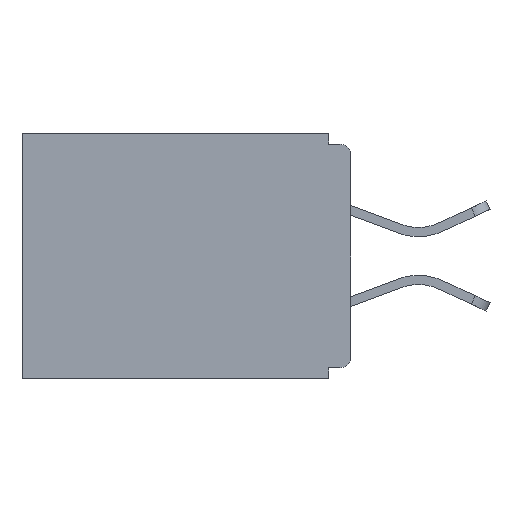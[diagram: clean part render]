
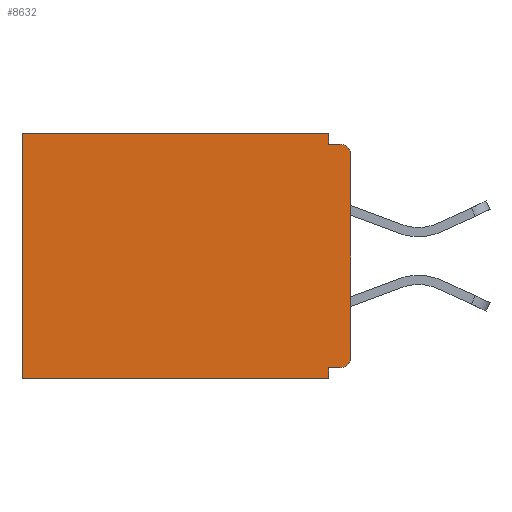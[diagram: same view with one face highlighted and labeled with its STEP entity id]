
A CAD part, left-side view. The second image highlights one B-rep face of the part: STEP entity #8632.
In plain terms, the highlighted planar face has unit normal (-1, 0, 0).
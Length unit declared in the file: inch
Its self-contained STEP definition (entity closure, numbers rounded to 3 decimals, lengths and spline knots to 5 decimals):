
#138 = ORIENTED_EDGE ( 'NONE', *, *, #10207, .T. ) ;
#171 = ORIENTED_EDGE ( 'NONE', *, *, #9532, .F. ) ;
#296 = VERTEX_POINT ( 'NONE', #675 ) ;
#557 = CARTESIAN_POINT ( 'NONE',  ( 0.298, 0.031, -0.343 ) ) ;
#586 = VERTEX_POINT ( 'NONE', #12412 ) ;
#630 = CARTESIAN_POINT ( 'NONE',  ( 0.298, 0., 0. ) ) ;
#675 = CARTESIAN_POINT ( 'NONE',  ( 0.298, 0.031, -0.015 ) ) ;
#912 = DIRECTION ( 'NONE',  ( 0., 0., -1. ) ) ;
#1182 = ORIENTED_EDGE ( 'NONE', *, *, #7727, .F. ) ;
#1664 = CARTESIAN_POINT ( 'NONE',  ( 0.298, 0.46, -0.343 ) ) ;
#2041 = LINE ( 'NONE', #21760, #22051 ) ;
#2055 = DIRECTION ( 'NONE',  ( 0., 0., -1. ) ) ;
#2333 = LINE ( 'NONE', #630, #8877 ) ;
#3120 = CARTESIAN_POINT ( 'NONE',  ( 0.298, 0.031, -0.328 ) ) ;
#3398 = EDGE_CURVE ( 'NONE', #586, #15834, #2333, .T. ) ;
#3418 = VECTOR ( 'NONE', #17324, 39.37008 ) ;
#4227 = DIRECTION ( 'NONE',  ( 1., 0., 0. ) ) ;
#4353 = CARTESIAN_POINT ( 'NONE',  ( 0.298, 0.015, -0.015 ) ) ;
#4906 = DIRECTION ( 'NONE',  ( 0., 1., 0. ) ) ;
#5036 = DIRECTION ( 'NONE',  ( 0., 0., -1. ) ) ;
#5037 = EDGE_LOOP ( 'NONE', ( #9502, #1182, #171, #5314, #21436, #9391, #26873, #21410, #138, #26231 ) ) ;
#5159 = LINE ( 'NONE', #25268, #23844 ) ;
#5314 = ORIENTED_EDGE ( 'NONE', *, *, #3398, .T. ) ;
#5332 = CARTESIAN_POINT ( 'NONE',  ( 0.298, 0.015, -0.03 ) ) ;
#5426 = DIRECTION ( 'NONE',  ( 0., 0., -1. ) ) ;
#5631 = LINE ( 'NONE', #20856, #14782 ) ;
#5661 = VERTEX_POINT ( 'NONE', #8861 ) ;
#5703 = VECTOR ( 'NONE', #12329, 39.37008 ) ;
#5867 = CARTESIAN_POINT ( 'NONE',  ( 0.298, 0.031, -0.343 ) ) ;
#6515 = PLANE ( 'NONE',  #23701 ) ;
#6704 = LINE ( 'NONE', #10229, #5703 ) ;
#7325 = CARTESIAN_POINT ( 'NONE',  ( 0.298, 0.46, 0. ) ) ;
#7727 = EDGE_CURVE ( 'NONE', #296, #10814, #6704, .T. ) ;
#8428 = CARTESIAN_POINT ( 'NONE',  ( 0.298, 0., 0. ) ) ;
#8632 = ADVANCED_FACE ( 'NONE', ( #12857 ), #6515, .F. ) ;
#8812 = VECTOR ( 'NONE', #17844, 39.37008 ) ;
#8861 = CARTESIAN_POINT ( 'NONE',  ( 0.298, 0., -0.03 ) ) ;
#8877 = VECTOR ( 'NONE', #9243, 39.37008 ) ;
#9243 = DIRECTION ( 'NONE',  ( 0., 1., 0. ) ) ;
#9391 = ORIENTED_EDGE ( 'NONE', *, *, #20432, .F. ) ;
#9502 = ORIENTED_EDGE ( 'NONE', *, *, #21094, .T. ) ;
#9532 = EDGE_CURVE ( 'NONE', #586, #296, #25723, .T. ) ;
#10207 = EDGE_CURVE ( 'NONE', #10832, #21256, #23380, .T. ) ;
#10229 = CARTESIAN_POINT ( 'NONE',  ( 0.298, 0., -0.015 ) ) ;
#10814 = VERTEX_POINT ( 'NONE', #4353 ) ;
#10832 = VERTEX_POINT ( 'NONE', #25603 ) ;
#11586 = EDGE_CURVE ( 'NONE', #5661, #21256, #5631, .T. ) ;
#12127 = AXIS2_PLACEMENT_3D ( 'NONE', #20993, #12805, #23366 ) ;
#12329 = DIRECTION ( 'NONE',  ( 0., -1., 0. ) ) ;
#12412 = CARTESIAN_POINT ( 'NONE',  ( 0.298, 0.031, 0. ) ) ;
#12618 = DIRECTION ( 'NONE',  ( 0., 0., -1. ) ) ;
#12805 = DIRECTION ( 'NONE',  ( -1., 0., 0. ) ) ;
#12857 = FACE_OUTER_BOUND ( 'NONE', #5037, .T. ) ;
#13257 = VERTEX_POINT ( 'NONE', #1664 ) ;
#14782 = VECTOR ( 'NONE', #2055, 39.37008 ) ;
#14915 = AXIS2_PLACEMENT_3D ( 'NONE', #5332, #22206, #5426 ) ;
#15834 = VERTEX_POINT ( 'NONE', #22258 ) ;
#16165 = EDGE_CURVE ( 'NONE', #15834, #13257, #23867, .T. ) ;
#17324 = DIRECTION ( 'NONE',  ( 0., 0., -1. ) ) ;
#17844 = DIRECTION ( 'NONE',  ( 0., 1., 0. ) ) ;
#18029 = CARTESIAN_POINT ( 'NONE',  ( 0.298, 0., -0.328 ) ) ;
#19620 = VERTEX_POINT ( 'NONE', #5867 ) ;
#20432 = EDGE_CURVE ( 'NONE', #19620, #13257, #2041, .T. ) ;
#20856 = CARTESIAN_POINT ( 'NONE',  ( 0.298, 0., 0. ) ) ;
#20939 = VECTOR ( 'NONE', #912, 39.37008 ) ;
#20993 = CARTESIAN_POINT ( 'NONE',  ( 0.298, 0.015, -0.313 ) ) ;
#21094 = EDGE_CURVE ( 'NONE', #5661, #10814, #22001, .T. ) ;
#21256 = VERTEX_POINT ( 'NONE', #25522 ) ;
#21410 = ORIENTED_EDGE ( 'NONE', *, *, #25514, .F. ) ;
#21436 = ORIENTED_EDGE ( 'NONE', *, *, #16165, .T. ) ;
#21760 = CARTESIAN_POINT ( 'NONE',  ( 0.298, 0., -0.343 ) ) ;
#22001 = CIRCLE ( 'NONE', #14915, 0.015 ) ;
#22051 = VECTOR ( 'NONE', #4906, 39.37008 ) ;
#22206 = DIRECTION ( 'NONE',  ( -1., 0., 0. ) ) ;
#22258 = CARTESIAN_POINT ( 'NONE',  ( 0.298, 0.46, 0. ) ) ;
#23366 = DIRECTION ( 'NONE',  ( 0., 0., -1. ) ) ;
#23380 = CIRCLE ( 'NONE', #12127, 0.015 ) ;
#23701 = AXIS2_PLACEMENT_3D ( 'NONE', #8428, #4227, #12618 ) ;
#23844 = VECTOR ( 'NONE', #5036, 39.37008 ) ;
#23867 = LINE ( 'NONE', #7325, #20939 ) ;
#24126 = VERTEX_POINT ( 'NONE', #3120 ) ;
#25268 = CARTESIAN_POINT ( 'NONE',  ( 0.298, 0.031, -0.343 ) ) ;
#25514 = EDGE_CURVE ( 'NONE', #10832, #24126, #26843, .T. ) ;
#25522 = CARTESIAN_POINT ( 'NONE',  ( 0.298, 0., -0.313 ) ) ;
#25603 = CARTESIAN_POINT ( 'NONE',  ( 0.298, 0.015, -0.328 ) ) ;
#25723 = LINE ( 'NONE', #557, #3418 ) ;
#26231 = ORIENTED_EDGE ( 'NONE', *, *, #11586, .F. ) ;
#26613 = EDGE_CURVE ( 'NONE', #24126, #19620, #5159, .T. ) ;
#26843 = LINE ( 'NONE', #18029, #8812 ) ;
#26873 = ORIENTED_EDGE ( 'NONE', *, *, #26613, .F. ) ;
